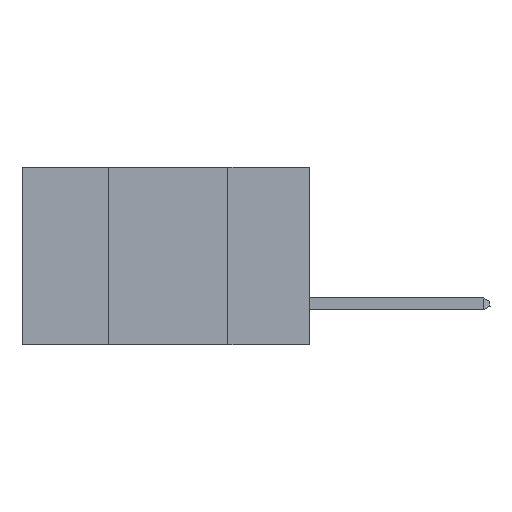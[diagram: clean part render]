
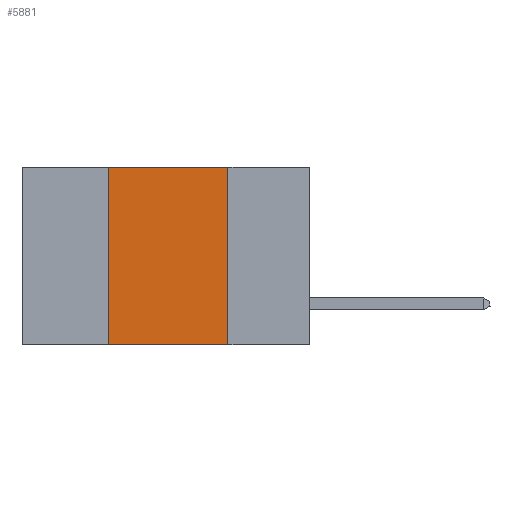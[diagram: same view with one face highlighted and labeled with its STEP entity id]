
A CAD part, left-side view. The second image highlights one B-rep face of the part: STEP entity #5881.
In plain terms, the highlighted planar face has unit normal (-1, 0, 0).
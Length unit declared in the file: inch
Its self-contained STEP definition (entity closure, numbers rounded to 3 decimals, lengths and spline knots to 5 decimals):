
#910 = CARTESIAN_POINT ( 'NONE',  ( 0., 0.6, 0. ) ) ;
#1060 = ORIENTED_EDGE ( 'NONE', *, *, #7650, .F. ) ;
#2423 = EDGE_CURVE ( 'NONE', #8550, #5561, #12143, .T. ) ;
#2450 = VERTEX_POINT ( 'NONE', #6359 ) ;
#2473 = PLANE ( 'NONE',  #5179 ) ;
#3106 = DIRECTION ( 'NONE',  ( 0., -1., 0. ) ) ;
#3188 = CARTESIAN_POINT ( 'NONE',  ( 0., 0.42, 0. ) ) ;
#3809 = VECTOR ( 'NONE', #9620, 39.37008 ) ;
#4188 = ORIENTED_EDGE ( 'NONE', *, *, #10157, .F. ) ;
#5179 = AXIS2_PLACEMENT_3D ( 'NONE', #10654, #8493, #10706 ) ;
#5486 = EDGE_CURVE ( 'NONE', #2450, #5561, #9210, .T. ) ;
#5561 = VERTEX_POINT ( 'NONE', #5904 ) ;
#5881 = ADVANCED_FACE ( 'NONE', ( #6961 ), #2473, .F. ) ;
#5904 = CARTESIAN_POINT ( 'NONE',  ( 0., 0.17, -0.37 ) ) ;
#6266 = ORIENTED_EDGE ( 'NONE', *, *, #2423, .T. ) ;
#6359 = CARTESIAN_POINT ( 'NONE',  ( 0., 0.17, 0. ) ) ;
#6686 = LINE ( 'NONE', #3188, #8283 ) ;
#6961 = FACE_OUTER_BOUND ( 'NONE', #7177, .T. ) ;
#7086 = ORIENTED_EDGE ( 'NONE', *, *, #5486, .F. ) ;
#7177 = EDGE_LOOP ( 'NONE', ( #7086, #1060, #4188, #6266 ) ) ;
#7216 = LINE ( 'NONE', #910, #10238 ) ;
#7650 = EDGE_CURVE ( 'NONE', #9174, #2450, #7216, .T. ) ;
#8283 = VECTOR ( 'NONE', #9246, 39.37008 ) ;
#8493 = DIRECTION ( 'NONE',  ( 1., 0., 0. ) ) ;
#8550 = VERTEX_POINT ( 'NONE', #9313 ) ;
#8727 = CARTESIAN_POINT ( 'NONE',  ( 0., 0.6, -0.37 ) ) ;
#9174 = VERTEX_POINT ( 'NONE', #11414 ) ;
#9210 = LINE ( 'NONE', #12632, #3809 ) ;
#9246 = DIRECTION ( 'NONE',  ( 0., 0., 1. ) ) ;
#9313 = CARTESIAN_POINT ( 'NONE',  ( 0., 0.42, -0.37 ) ) ;
#9620 = DIRECTION ( 'NONE',  ( 0., 0., -1. ) ) ;
#10157 = EDGE_CURVE ( 'NONE', #8550, #9174, #6686, .T. ) ;
#10238 = VECTOR ( 'NONE', #12086, 39.37008 ) ;
#10654 = CARTESIAN_POINT ( 'NONE',  ( 0., 0.6, 0. ) ) ;
#10706 = DIRECTION ( 'NONE',  ( 0., 0., -1. ) ) ;
#11414 = CARTESIAN_POINT ( 'NONE',  ( 0., 0.42, 0. ) ) ;
#12086 = DIRECTION ( 'NONE',  ( 0., -1., 0. ) ) ;
#12143 = LINE ( 'NONE', #8727, #12447 ) ;
#12447 = VECTOR ( 'NONE', #3106, 39.37008 ) ;
#12632 = CARTESIAN_POINT ( 'NONE',  ( 0., 0.17, 0. ) ) ;
